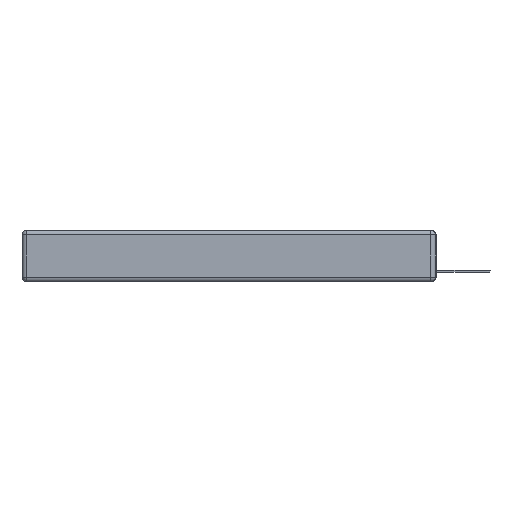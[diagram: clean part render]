
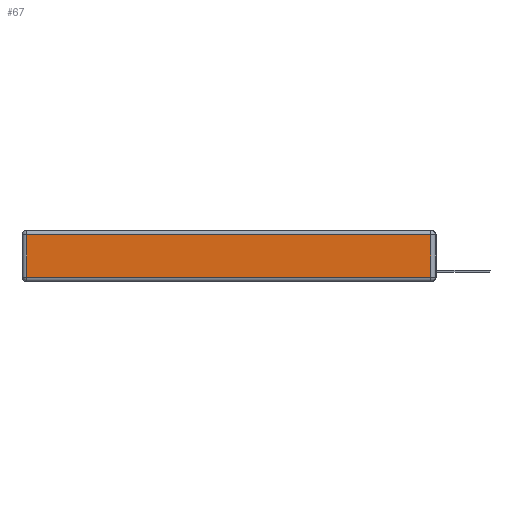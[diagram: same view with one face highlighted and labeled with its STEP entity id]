
A CAD part, left-side view. The second image highlights one B-rep face of the part: STEP entity #67.
In plain terms, the highlighted planar face has unit normal (-1, 0, 0).
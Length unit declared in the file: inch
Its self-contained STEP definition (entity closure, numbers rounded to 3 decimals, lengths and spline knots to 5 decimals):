
#67 = ADVANCED_FACE ( 'NONE', ( #5859 ), #8906, .T. ) ;
#97 = CARTESIAN_POINT ( 'NONE',  ( 0., 2.72, -0.03 ) ) ;
#531 = CARTESIAN_POINT ( 'NONE',  ( 0., 2.72, -0.343 ) ) ;
#1657 = CARTESIAN_POINT ( 'NONE',  ( 0., 0., -0.313 ) ) ;
#1961 = ORIENTED_EDGE ( 'NONE', *, *, #3429, .T. ) ;
#2618 = DIRECTION ( 'NONE',  ( 0., 1., 0. ) ) ;
#2940 = EDGE_CURVE ( 'NONE', #3885, #4232, #14791, .T. ) ;
#3104 = LINE ( 'NONE', #1657, #13661 ) ;
#3429 = EDGE_CURVE ( 'NONE', #4232, #16435, #3104, .T. ) ;
#3885 = VERTEX_POINT ( 'NONE', #97 ) ;
#4232 = VERTEX_POINT ( 'NONE', #11971 ) ;
#4499 = DIRECTION ( 'NONE',  ( 0., 0., 1. ) ) ;
#5311 = LINE ( 'NONE', #11144, #9703 ) ;
#5859 = FACE_OUTER_BOUND ( 'NONE', #13431, .T. ) ;
#7329 = EDGE_CURVE ( 'NONE', #7383, #3885, #15549, .T. ) ;
#7383 = VERTEX_POINT ( 'NONE', #17165 ) ;
#8196 = CARTESIAN_POINT ( 'NONE',  ( 0., 2.75, -0.03 ) ) ;
#8635 = DIRECTION ( 'NONE',  ( -1., 0., 0. ) ) ;
#8811 = CARTESIAN_POINT ( 'NONE',  ( 0., 0., -0.343 ) ) ;
#8906 = PLANE ( 'NONE',  #8980 ) ;
#8980 = AXIS2_PLACEMENT_3D ( 'NONE', #8811, #8635, #4499 ) ;
#9519 = DIRECTION ( 'NONE',  ( 0., 0., 1. ) ) ;
#9703 = VECTOR ( 'NONE', #9519, 39.37008 ) ;
#10474 = DIRECTION ( 'NONE',  ( 0., -1., 0. ) ) ;
#11144 = CARTESIAN_POINT ( 'NONE',  ( 0., 0.03, -0.343 ) ) ;
#11930 = ORIENTED_EDGE ( 'NONE', *, *, #2940, .T. ) ;
#11971 = CARTESIAN_POINT ( 'NONE',  ( 0., 2.72, -0.313 ) ) ;
#12497 = VECTOR ( 'NONE', #2618, 39.37008 ) ;
#13431 = EDGE_LOOP ( 'NONE', ( #1961, #16703, #13847, #11930 ) ) ;
#13468 = DIRECTION ( 'NONE',  ( 0., 0., -1. ) ) ;
#13661 = VECTOR ( 'NONE', #10474, 39.37008 ) ;
#13847 = ORIENTED_EDGE ( 'NONE', *, *, #7329, .T. ) ;
#14085 = VECTOR ( 'NONE', #13468, 39.37008 ) ;
#14791 = LINE ( 'NONE', #531, #14085 ) ;
#15483 = EDGE_CURVE ( 'NONE', #16435, #7383, #5311, .T. ) ;
#15549 = LINE ( 'NONE', #8196, #12497 ) ;
#16435 = VERTEX_POINT ( 'NONE', #17367 ) ;
#16703 = ORIENTED_EDGE ( 'NONE', *, *, #15483, .T. ) ;
#17165 = CARTESIAN_POINT ( 'NONE',  ( 0., 0.03, -0.03 ) ) ;
#17367 = CARTESIAN_POINT ( 'NONE',  ( 0., 0.03, -0.313 ) ) ;
